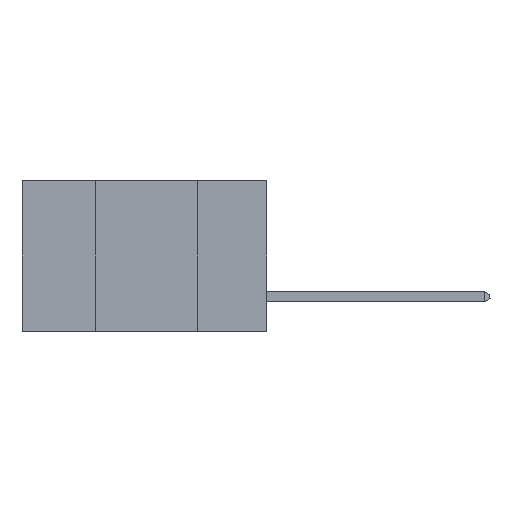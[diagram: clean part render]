
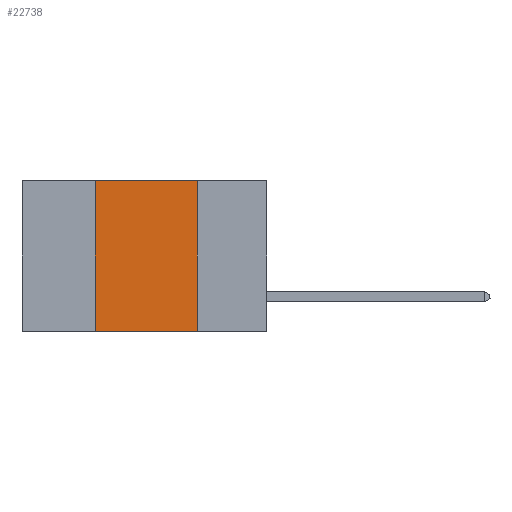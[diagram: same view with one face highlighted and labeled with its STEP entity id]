
A CAD part, left-side view. The second image highlights one B-rep face of the part: STEP entity #22738.
In plain terms, the highlighted planar face has unit normal (-1, 0, 0).
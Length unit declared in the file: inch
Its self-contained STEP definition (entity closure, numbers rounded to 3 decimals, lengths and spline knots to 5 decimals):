
#2493 = ORIENTED_EDGE ( 'NONE', *, *, #21499, .T. ) ;
#3834 = PLANE ( 'NONE',  #7191 ) ;
#4389 = CARTESIAN_POINT ( 'NONE',  ( 0., 0.42, 0. ) ) ;
#4510 = CARTESIAN_POINT ( 'NONE',  ( 0., 0.6, -0.37 ) ) ;
#7181 = EDGE_LOOP ( 'NONE', ( #16978, #19302, #24205, #2493 ) ) ;
#7191 = AXIS2_PLACEMENT_3D ( 'NONE', #18883, #7667, #20741 ) ;
#7628 = VECTOR ( 'NONE', #23116, 39.37008 ) ;
#7667 = DIRECTION ( 'NONE',  ( 1., 0., 0. ) ) ;
#8252 = CARTESIAN_POINT ( 'NONE',  ( 0., 0.6, 0. ) ) ;
#10267 = VECTOR ( 'NONE', #15778, 39.37008 ) ;
#11357 = VERTEX_POINT ( 'NONE', #16808 ) ;
#11955 = DIRECTION ( 'NONE',  ( 0., 0., 1. ) ) ;
#12778 = EDGE_CURVE ( 'NONE', #18586, #21588, #15272, .T. ) ;
#13169 = LINE ( 'NONE', #8252, #7628 ) ;
#13568 = EDGE_CURVE ( 'NONE', #21588, #11357, #13169, .T. ) ;
#14134 = CARTESIAN_POINT ( 'NONE',  ( 0., 0.42, 0. ) ) ;
#14699 = VECTOR ( 'NONE', #11955, 39.37008 ) ;
#15083 = VECTOR ( 'NONE', #17635, 39.37008 ) ;
#15272 = LINE ( 'NONE', #4389, #14699 ) ;
#15678 = LINE ( 'NONE', #15731, #15083 ) ;
#15731 = CARTESIAN_POINT ( 'NONE',  ( 0., 0.17, 0. ) ) ;
#15778 = DIRECTION ( 'NONE',  ( 0., -1., 0. ) ) ;
#16390 = LINE ( 'NONE', #4510, #10267 ) ;
#16808 = CARTESIAN_POINT ( 'NONE',  ( 0., 0.17, 0. ) ) ;
#16978 = ORIENTED_EDGE ( 'NONE', *, *, #23578, .F. ) ;
#17635 = DIRECTION ( 'NONE',  ( 0., 0., -1. ) ) ;
#18586 = VERTEX_POINT ( 'NONE', #22056 ) ;
#18883 = CARTESIAN_POINT ( 'NONE',  ( 0., 0.6, 0. ) ) ;
#19302 = ORIENTED_EDGE ( 'NONE', *, *, #13568, .F. ) ;
#20693 = FACE_OUTER_BOUND ( 'NONE', #7181, .T. ) ;
#20741 = DIRECTION ( 'NONE',  ( 0., 0., -1. ) ) ;
#21028 = VERTEX_POINT ( 'NONE', #21906 ) ;
#21499 = EDGE_CURVE ( 'NONE', #18586, #21028, #16390, .T. ) ;
#21588 = VERTEX_POINT ( 'NONE', #14134 ) ;
#21906 = CARTESIAN_POINT ( 'NONE',  ( 0., 0.17, -0.37 ) ) ;
#22056 = CARTESIAN_POINT ( 'NONE',  ( 0., 0.42, -0.37 ) ) ;
#22738 = ADVANCED_FACE ( 'NONE', ( #20693 ), #3834, .F. ) ;
#23116 = DIRECTION ( 'NONE',  ( 0., -1., 0. ) ) ;
#23578 = EDGE_CURVE ( 'NONE', #11357, #21028, #15678, .T. ) ;
#24205 = ORIENTED_EDGE ( 'NONE', *, *, #12778, .F. ) ;
